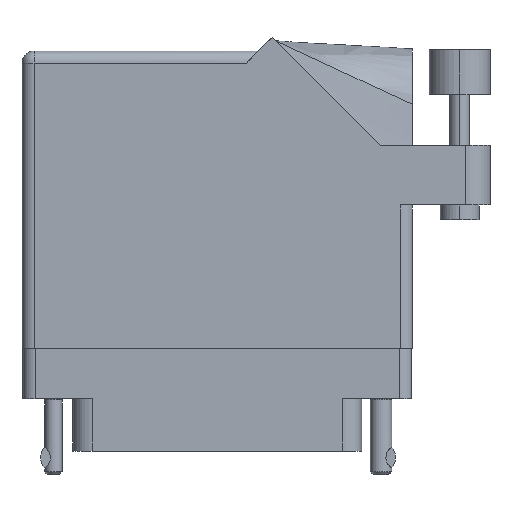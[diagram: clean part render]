
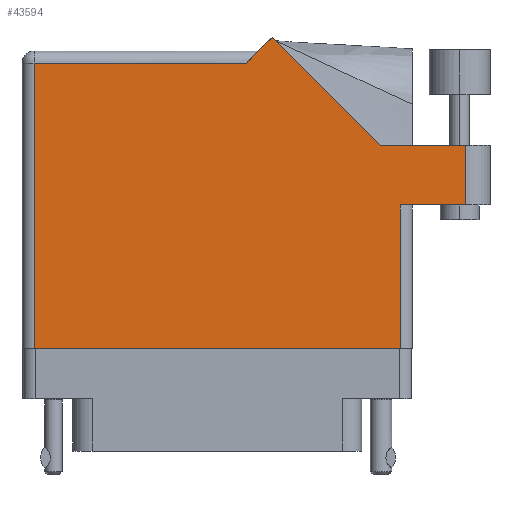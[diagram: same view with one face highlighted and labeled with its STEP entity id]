
A CAD part, front view. The second image highlights one B-rep face of the part: STEP entity #43594.
In plain terms, the highlighted face is planar.
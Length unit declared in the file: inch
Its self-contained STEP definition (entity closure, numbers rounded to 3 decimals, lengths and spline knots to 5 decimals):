
#274 = LINE ( 'NONE', #33238, #9552 ) ;
#352 = CARTESIAN_POINT ( 'NONE',  ( 1.84442, 1.044, 0. ) ) ;
#684 = ORIENTED_EDGE ( 'NONE', *, *, #44240, .T. ) ;
#716 = CARTESIAN_POINT ( 'NONE',  ( 0., 1.53, 0. ) ) ;
#1584 = DIRECTION ( 'NONE',  ( 0., -1., 0. ) ) ;
#1760 = VECTOR ( 'NONE', #23082, 39.37008 ) ;
#1762 = ORIENTED_EDGE ( 'NONE', *, *, #37049, .T. ) ;
#1813 = CARTESIAN_POINT ( 'NONE',  ( 0., 1.468, 0. ) ) ;
#2001 = CARTESIAN_POINT ( 'NONE',  ( 2.41, 1.044, 0. ) ) ;
#4791 = VECTOR ( 'NONE', #43696, 39.37008 ) ;
#5632 = ORIENTED_EDGE ( 'NONE', *, *, #13084, .T. ) ;
#6172 = DIRECTION ( 'NONE',  ( 0., 1., 0. ) ) ;
#6941 = DIRECTION ( 'NONE',  ( -0.707, 0.707, 0. ) ) ;
#6947 = LINE ( 'NONE', #22988, #23112 ) ;
#7186 = VERTEX_POINT ( 'NONE', #28117 ) ;
#7645 = ORIENTED_EDGE ( 'NONE', *, *, #24782, .T. ) ;
#8265 = CARTESIAN_POINT ( 'NONE',  ( 1.155, 1.468, 0. ) ) ;
#8305 = DIRECTION ( 'NONE',  ( -1., 0., 0. ) ) ;
#8766 = EDGE_CURVE ( 'NONE', #43652, #7186, #6947, .T. ) ;
#9552 = VECTOR ( 'NONE', #48074, 39.37008 ) ;
#10468 = CARTESIAN_POINT ( 'NONE',  ( 0.062, 0., 0. ) ) ;
#10757 = EDGE_CURVE ( 'NONE', #44929, #20327, #26283, .T. ) ;
#13019 = VERTEX_POINT ( 'NONE', #30608 ) ;
#13084 = EDGE_CURVE ( 'NONE', #20327, #43652, #28397, .T. ) ;
#14853 = CARTESIAN_POINT ( 'NONE',  ( 2.285, 1.044, 0. ) ) ;
#15109 = LINE ( 'NONE', #14853, #4791 ) ;
#15166 = VECTOR ( 'NONE', #16893, 39.37008 ) ;
#15591 = FACE_OUTER_BOUND ( 'NONE', #18840, .T. ) ;
#16893 = DIRECTION ( 'NONE',  ( -1., 0., 0. ) ) ;
#17432 = EDGE_CURVE ( 'NONE', #13019, #22937, #41090, .T. ) ;
#17930 = DIRECTION ( 'NONE',  ( 1., 0., 0. ) ) ;
#18840 = EDGE_LOOP ( 'NONE', ( #29647, #35473, #45029, #31736, #1762, #684, #7645, #31101, #5632 ) ) ;
#20327 = VERTEX_POINT ( 'NONE', #37622 ) ;
#20342 = VECTOR ( 'NONE', #45733, 39.37008 ) ;
#21229 = VECTOR ( 'NONE', #6172, 39.37008 ) ;
#22699 = PLANE ( 'NONE',  #29103 ) ;
#22937 = VERTEX_POINT ( 'NONE', #37797 ) ;
#22954 = DIRECTION ( 'NONE',  ( 0., 0., -1. ) ) ;
#22988 = CARTESIAN_POINT ( 'NONE',  ( 2.01, 0.737, 0. ) ) ;
#23082 = DIRECTION ( 'NONE',  ( -1., 0., 0. ) ) ;
#23112 = VECTOR ( 'NONE', #17930, 39.37008 ) ;
#24002 = CARTESIAN_POINT ( 'NONE',  ( 1.948, 0.737, 0. ) ) ;
#24782 = EDGE_CURVE ( 'NONE', #47858, #44929, #35281, .T. ) ;
#26283 = LINE ( 'NONE', #41136, #20342 ) ;
#26428 = CARTESIAN_POINT ( 'NONE',  ( 0.062, 1.468, 0. ) ) ;
#28117 = CARTESIAN_POINT ( 'NONE',  ( 2.285, 0.737, 0. ) ) ;
#28397 = LINE ( 'NONE', #24002, #21229 ) ;
#29103 = AXIS2_PLACEMENT_3D ( 'NONE', #716, #22954, #8305 ) ;
#29647 = ORIENTED_EDGE ( 'NONE', *, *, #8766, .T. ) ;
#30608 = CARTESIAN_POINT ( 'NONE',  ( 1.84442, 1.044, 0. ) ) ;
#31101 = ORIENTED_EDGE ( 'NONE', *, *, #10757, .T. ) ;
#31736 = ORIENTED_EDGE ( 'NONE', *, *, #17432, .T. ) ;
#33238 = CARTESIAN_POINT ( 'NONE',  ( 1.217, 1.53, 0. ) ) ;
#34277 = LINE ( 'NONE', #1813, #1760 ) ;
#34485 = VECTOR ( 'NONE', #6941, 39.37008 ) ;
#34865 = VERTEX_POINT ( 'NONE', #8265 ) ;
#35281 = LINE ( 'NONE', #35762, #43844 ) ;
#35473 = ORIENTED_EDGE ( 'NONE', *, *, #41716, .T. ) ;
#35762 = CARTESIAN_POINT ( 'NONE',  ( 0.062, 0., 0. ) ) ;
#36156 = LINE ( 'NONE', #2001, #15166 ) ;
#37049 = EDGE_CURVE ( 'NONE', #22937, #34865, #274, .T. ) ;
#37622 = CARTESIAN_POINT ( 'NONE',  ( 1.948, 0., 0. ) ) ;
#37797 = CARTESIAN_POINT ( 'NONE',  ( 1.28771, 1.60071, 0. ) ) ;
#38934 = EDGE_CURVE ( 'NONE', #44685, #13019, #36156, .T. ) ;
#41090 = LINE ( 'NONE', #352, #34485 ) ;
#41136 = CARTESIAN_POINT ( 'NONE',  ( 0., 0., 0. ) ) ;
#41221 = CARTESIAN_POINT ( 'NONE',  ( 1.948, 0.737, 0. ) ) ;
#41285 = CARTESIAN_POINT ( 'NONE',  ( 2.285, 1.044, 0. ) ) ;
#41716 = EDGE_CURVE ( 'NONE', #7186, #44685, #15109, .T. ) ;
#43594 = ADVANCED_FACE ( 'NONE', ( #15591 ), #22699, .F. ) ;
#43652 = VERTEX_POINT ( 'NONE', #41221 ) ;
#43696 = DIRECTION ( 'NONE',  ( 0., 1., 0. ) ) ;
#43844 = VECTOR ( 'NONE', #1584, 39.37008 ) ;
#44240 = EDGE_CURVE ( 'NONE', #34865, #47858, #34277, .T. ) ;
#44685 = VERTEX_POINT ( 'NONE', #41285 ) ;
#44929 = VERTEX_POINT ( 'NONE', #10468 ) ;
#45029 = ORIENTED_EDGE ( 'NONE', *, *, #38934, .T. ) ;
#45733 = DIRECTION ( 'NONE',  ( 1., 0., 0. ) ) ;
#47858 = VERTEX_POINT ( 'NONE', #26428 ) ;
#48074 = DIRECTION ( 'NONE',  ( -0.707, -0.707, 0. ) ) ;
